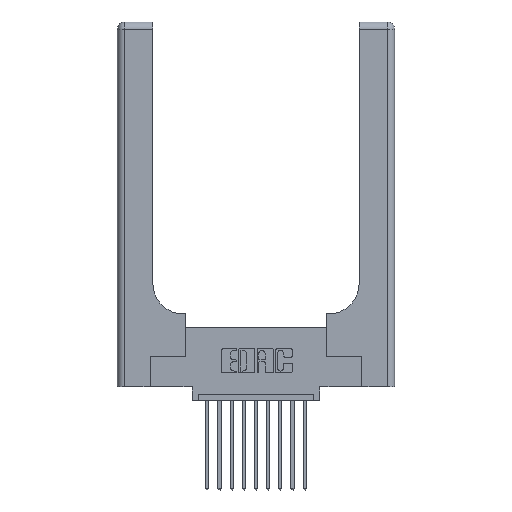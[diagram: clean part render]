
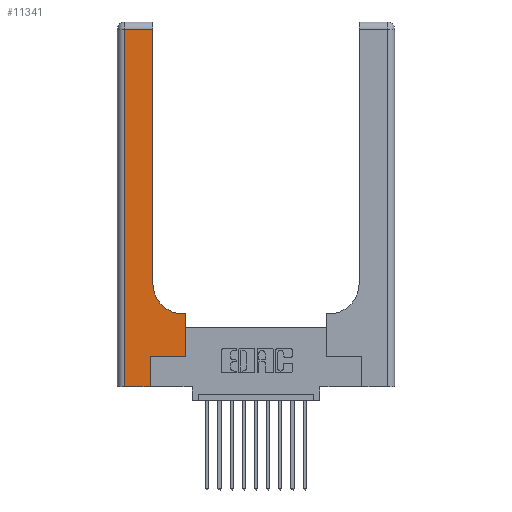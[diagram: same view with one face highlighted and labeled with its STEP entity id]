
A CAD part, top view. The second image highlights one B-rep face of the part: STEP entity #11341.
In plain terms, the highlighted planar face has unit normal (0, 0, 1).
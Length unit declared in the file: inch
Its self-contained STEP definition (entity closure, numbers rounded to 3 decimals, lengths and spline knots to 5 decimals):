
#363 = LINE ( 'NONE', #5351, #5509 ) ;
#383 = ORIENTED_EDGE ( 'NONE', *, *, #4048, .T. ) ;
#1039 = VECTOR ( 'NONE', #14425, 39.37008 ) ;
#1309 = CARTESIAN_POINT ( 'NONE',  ( 0.2915, 0.6, 0.37 ) ) ;
#1503 = VECTOR ( 'NONE', #5043, 39.37008 ) ;
#1710 = EDGE_CURVE ( 'NONE', #16237, #9972, #5100, .T. ) ;
#1838 = LINE ( 'NONE', #5684, #14659 ) ;
#1851 = LINE ( 'NONE', #13261, #5450 ) ;
#2021 = LINE ( 'NONE', #14817, #9441 ) ;
#2150 = CARTESIAN_POINT ( 'NONE',  ( 0.269, 0.25, 0.37 ) ) ;
#3498 = EDGE_CURVE ( 'NONE', #4517, #11811, #1851, .T. ) ;
#3620 = CARTESIAN_POINT ( 'NONE',  ( 0.5585, 0.6, 0.37 ) ) ;
#3636 = DIRECTION ( 'NONE',  ( 1., 0., 0. ) ) ;
#3638 = CARTESIAN_POINT ( 'NONE',  ( 0.2915, 0.85, 0.37 ) ) ;
#3643 = EDGE_CURVE ( 'NONE', #14835, #16237, #15084, .T. ) ;
#4048 = EDGE_CURVE ( 'NONE', #16323, #15574, #1838, .T. ) ;
#4051 = EDGE_CURVE ( 'NONE', #9972, #13676, #9439, .T. ) ;
#4244 = FACE_OUTER_BOUND ( 'NONE', #12114, .T. ) ;
#4479 = CARTESIAN_POINT ( 'NONE',  ( 0.06, 2.94, 0.37 ) ) ;
#4517 = VERTEX_POINT ( 'NONE', #15117 ) ;
#4762 = EDGE_CURVE ( 'NONE', #15574, #4517, #2021, .T. ) ;
#5043 = DIRECTION ( 'NONE',  ( -1., 0., 0. ) ) ;
#5100 = CIRCLE ( 'NONE', #11153, 0.25 ) ;
#5351 = CARTESIAN_POINT ( 'NONE',  ( 0., 2.94, 0.37 ) ) ;
#5450 = VECTOR ( 'NONE', #9913, 39.37008 ) ;
#5468 = DIRECTION ( 'NONE',  ( 0., -1., 0. ) ) ;
#5509 = VECTOR ( 'NONE', #6971, 39.37008 ) ;
#5684 = CARTESIAN_POINT ( 'NONE',  ( 0.06, 3., 0.37 ) ) ;
#6971 = DIRECTION ( 'NONE',  ( -1., 0., 0. ) ) ;
#7080 = CARTESIAN_POINT ( 'NONE',  ( 0.5585, 0.25, 0.37 ) ) ;
#7385 = ORIENTED_EDGE ( 'NONE', *, *, #3643, .T. ) ;
#7545 = PLANE ( 'NONE',  #9315 ) ;
#7724 = ORIENTED_EDGE ( 'NONE', *, *, #9217, .T. ) ;
#7914 = VECTOR ( 'NONE', #12095, 39.37008 ) ;
#8018 = VECTOR ( 'NONE', #8768, 39.37008 ) ;
#8432 = DIRECTION ( 'NONE',  ( 1., 0., 0. ) ) ;
#8436 = EDGE_CURVE ( 'NONE', #13676, #16323, #363, .T. ) ;
#8509 = ORIENTED_EDGE ( 'NONE', *, *, #12541, .T. ) ;
#8587 = CARTESIAN_POINT ( 'NONE',  ( 0.5415, 0.85, 0.37 ) ) ;
#8762 = DIRECTION ( 'NONE',  ( 0., 0., -1. ) ) ;
#8768 = DIRECTION ( 'NONE',  ( 1., 0., 0. ) ) ;
#9217 = EDGE_CURVE ( 'NONE', #10709, #14835, #9904, .T. ) ;
#9315 = AXIS2_PLACEMENT_3D ( 'NONE', #15151, #8762, #16506 ) ;
#9439 = LINE ( 'NONE', #13139, #1039 ) ;
#9441 = VECTOR ( 'NONE', #8432, 39.37008 ) ;
#9787 = ORIENTED_EDGE ( 'NONE', *, *, #3498, .T. ) ;
#9904 = LINE ( 'NONE', #10808, #7914 ) ;
#9913 = DIRECTION ( 'NONE',  ( 0., 1., 0. ) ) ;
#9972 = VERTEX_POINT ( 'NONE', #3638 ) ;
#10001 = DIRECTION ( 'NONE',  ( 0., 0., -1. ) ) ;
#10107 = ORIENTED_EDGE ( 'NONE', *, *, #8436, .T. ) ;
#10317 = ORIENTED_EDGE ( 'NONE', *, *, #4762, .T. ) ;
#10440 = ORIENTED_EDGE ( 'NONE', *, *, #1710, .T. ) ;
#10495 = ORIENTED_EDGE ( 'NONE', *, *, #4051, .T. ) ;
#10526 = CARTESIAN_POINT ( 'NONE',  ( 0.5415, 0.6, 0.37 ) ) ;
#10709 = VERTEX_POINT ( 'NONE', #7080 ) ;
#10808 = CARTESIAN_POINT ( 'NONE',  ( 0.5585, 0.25, 0.37 ) ) ;
#11153 = AXIS2_PLACEMENT_3D ( 'NONE', #8587, #10001, #3636 ) ;
#11178 = CARTESIAN_POINT ( 'NONE',  ( 0.269, 0.25, 0.37 ) ) ;
#11341 = ADVANCED_FACE ( 'NONE', ( #4244 ), #7545, .F. ) ;
#11811 = VERTEX_POINT ( 'NONE', #2150 ) ;
#12095 = DIRECTION ( 'NONE',  ( 0., 1., 0. ) ) ;
#12114 = EDGE_LOOP ( 'NONE', ( #10495, #10107, #383, #10317, #9787, #8509, #7724, #7385, #10440 ) ) ;
#12541 = EDGE_CURVE ( 'NONE', #11811, #10709, #15004, .T. ) ;
#13139 = CARTESIAN_POINT ( 'NONE',  ( 0.2915, 3., 0.37 ) ) ;
#13246 = CARTESIAN_POINT ( 'NONE',  ( 0.06, 0., 0.37 ) ) ;
#13261 = CARTESIAN_POINT ( 'NONE',  ( 0.269, 0., 0.37 ) ) ;
#13676 = VERTEX_POINT ( 'NONE', #15005 ) ;
#14425 = DIRECTION ( 'NONE',  ( 0., 1., 0. ) ) ;
#14659 = VECTOR ( 'NONE', #5468, 39.37008 ) ;
#14817 = CARTESIAN_POINT ( 'NONE',  ( 0., 0., 0.37 ) ) ;
#14835 = VERTEX_POINT ( 'NONE', #3620 ) ;
#15004 = LINE ( 'NONE', #11178, #8018 ) ;
#15005 = CARTESIAN_POINT ( 'NONE',  ( 0.2915, 2.94, 0.37 ) ) ;
#15084 = LINE ( 'NONE', #1309, #1503 ) ;
#15117 = CARTESIAN_POINT ( 'NONE',  ( 0.269, 0., 0.37 ) ) ;
#15151 = CARTESIAN_POINT ( 'NONE',  ( 0., 3., 0.37 ) ) ;
#15574 = VERTEX_POINT ( 'NONE', #13246 ) ;
#16237 = VERTEX_POINT ( 'NONE', #10526 ) ;
#16323 = VERTEX_POINT ( 'NONE', #4479 ) ;
#16506 = DIRECTION ( 'NONE',  ( -1., 0., 0. ) ) ;
